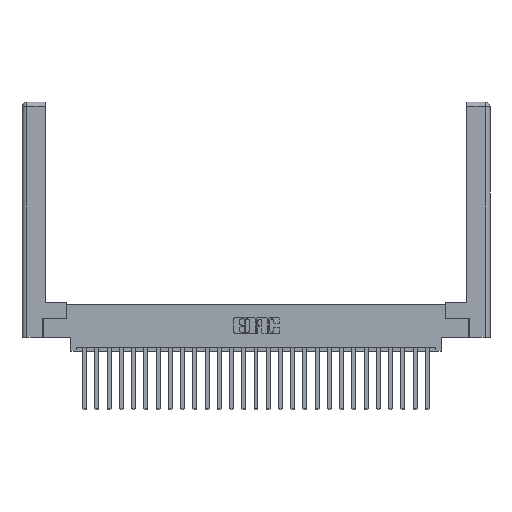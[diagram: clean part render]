
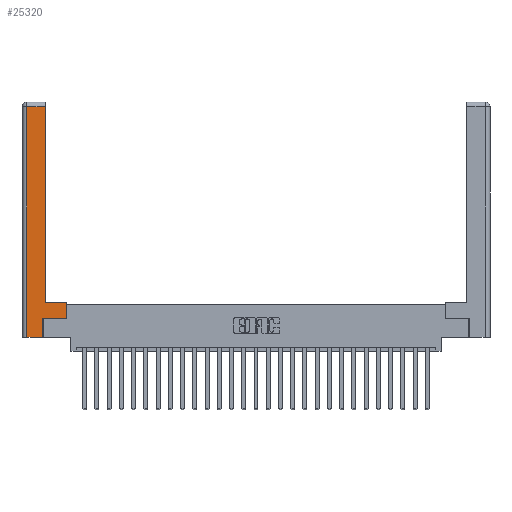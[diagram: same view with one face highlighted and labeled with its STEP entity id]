
A CAD part, top view. The second image highlights one B-rep face of the part: STEP entity #25320.
In plain terms, the highlighted planar face has unit normal (0, 0, 1).
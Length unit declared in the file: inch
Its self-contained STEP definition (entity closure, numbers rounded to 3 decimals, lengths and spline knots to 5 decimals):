
#181 = ORIENTED_EDGE ( 'NONE', *, *, #18120, .T. ) ;
#183 = CARTESIAN_POINT ( 'NONE',  ( 0.565, 0.245, 0. ) ) ;
#653 = LINE ( 'NONE', #11750, #4241 ) ;
#1042 = CARTESIAN_POINT ( 'NONE',  ( 0.265, 0., 0. ) ) ;
#1676 = LINE ( 'NONE', #9965, #18192 ) ;
#2169 = VERTEX_POINT ( 'NONE', #183 ) ;
#3119 = CARTESIAN_POINT ( 'NONE',  ( 0.295, 0.45, 0. ) ) ;
#4077 = ORIENTED_EDGE ( 'NONE', *, *, #25276, .T. ) ;
#4241 = VECTOR ( 'NONE', #21911, 39.37008 ) ;
#4750 = FACE_OUTER_BOUND ( 'NONE', #24954, .T. ) ;
#4895 = VECTOR ( 'NONE', #6860, 39.37008 ) ;
#5386 = CARTESIAN_POINT ( 'NONE',  ( 0.295, 0.45, 0. ) ) ;
#5561 = EDGE_CURVE ( 'NONE', #22152, #10963, #23265, .T. ) ;
#5761 = ORIENTED_EDGE ( 'NONE', *, *, #18331, .T. ) ;
#5882 = EDGE_CURVE ( 'NONE', #16050, #10681, #653, .T. ) ;
#6171 = VECTOR ( 'NONE', #11634, 39.37008 ) ;
#6860 = DIRECTION ( 'NONE',  ( 0., 1., 0. ) ) ;
#7297 = CARTESIAN_POINT ( 'NONE',  ( 0.265, 0.245, 0. ) ) ;
#7337 = ORIENTED_EDGE ( 'NONE', *, *, #5882, .T. ) ;
#7448 = VERTEX_POINT ( 'NONE', #13748 ) ;
#7829 = DIRECTION ( 'NONE',  ( 0., -1., 0. ) ) ;
#8129 = LINE ( 'NONE', #21230, #21371 ) ;
#8367 = AXIS2_PLACEMENT_3D ( 'NONE', #10323, #26649, #16479 ) ;
#8398 = DIRECTION ( 'NONE',  ( 1., 0., 0. ) ) ;
#8444 = CARTESIAN_POINT ( 'NONE',  ( 0.0615, 2.94, 0. ) ) ;
#9965 = CARTESIAN_POINT ( 'NONE',  ( 0.0615, 0., 0. ) ) ;
#10054 = PLANE ( 'NONE',  #8367 ) ;
#10323 = CARTESIAN_POINT ( 'NONE',  ( 0., 0., 0. ) ) ;
#10681 = VERTEX_POINT ( 'NONE', #16983 ) ;
#10720 = ORIENTED_EDGE ( 'NONE', *, *, #5561, .T. ) ;
#10963 = VERTEX_POINT ( 'NONE', #7297 ) ;
#11634 = DIRECTION ( 'NONE',  ( 0., 1., 0. ) ) ;
#11750 = CARTESIAN_POINT ( 'NONE',  ( 0.295, 3., 0. ) ) ;
#13748 = CARTESIAN_POINT ( 'NONE',  ( 0.0615, 0., 0. ) ) ;
#14403 = DIRECTION ( 'NONE',  ( -1., 0., 0. ) ) ;
#15169 = DIRECTION ( 'NONE',  ( 1., 0., 0. ) ) ;
#16050 = VERTEX_POINT ( 'NONE', #5386 ) ;
#16479 = DIRECTION ( 'NONE',  ( -1., 0., 0. ) ) ;
#16523 = CARTESIAN_POINT ( 'NONE',  ( 0.265, 0., 0. ) ) ;
#16851 = CARTESIAN_POINT ( 'NONE',  ( 0.0615, 2.94, 0. ) ) ;
#16983 = CARTESIAN_POINT ( 'NONE',  ( 0.295, 2.94, 0. ) ) ;
#17135 = CARTESIAN_POINT ( 'NONE',  ( 0.565, 0.45, 0. ) ) ;
#17183 = LINE ( 'NONE', #16523, #24277 ) ;
#17530 = VECTOR ( 'NONE', #26356, 39.37008 ) ;
#18120 = EDGE_CURVE ( 'NONE', #7448, #22152, #17183, .T. ) ;
#18161 = LINE ( 'NONE', #3119, #17530 ) ;
#18192 = VECTOR ( 'NONE', #7829, 39.37008 ) ;
#18331 = EDGE_CURVE ( 'NONE', #22255, #16050, #18161, .T. ) ;
#18707 = EDGE_CURVE ( 'NONE', #2169, #22255, #22301, .T. ) ;
#19498 = VECTOR ( 'NONE', #14403, 39.37008 ) ;
#19935 = CARTESIAN_POINT ( 'NONE',  ( 0.265, 0.245, 0. ) ) ;
#19993 = EDGE_CURVE ( 'NONE', #10681, #21200, #22020, .T. ) ;
#20684 = EDGE_CURVE ( 'NONE', #10963, #2169, #8129, .T. ) ;
#21200 = VERTEX_POINT ( 'NONE', #16851 ) ;
#21230 = CARTESIAN_POINT ( 'NONE',  ( 0.565, 0.245, 0. ) ) ;
#21371 = VECTOR ( 'NONE', #15169, 39.37008 ) ;
#21911 = DIRECTION ( 'NONE',  ( 0., 1., 0. ) ) ;
#22020 = LINE ( 'NONE', #8444, #19498 ) ;
#22152 = VERTEX_POINT ( 'NONE', #1042 ) ;
#22255 = VERTEX_POINT ( 'NONE', #23902 ) ;
#22301 = LINE ( 'NONE', #17135, #4895 ) ;
#23152 = ORIENTED_EDGE ( 'NONE', *, *, #19993, .T. ) ;
#23265 = LINE ( 'NONE', #19935, #6171 ) ;
#23902 = CARTESIAN_POINT ( 'NONE',  ( 0.565, 0.45, 0. ) ) ;
#24277 = VECTOR ( 'NONE', #8398, 39.37008 ) ;
#24361 = ORIENTED_EDGE ( 'NONE', *, *, #18707, .T. ) ;
#24954 = EDGE_LOOP ( 'NONE', ( #7337, #23152, #4077, #181, #10720, #26470, #24361, #5761 ) ) ;
#25276 = EDGE_CURVE ( 'NONE', #21200, #7448, #1676, .T. ) ;
#25320 = ADVANCED_FACE ( 'NONE', ( #4750 ), #10054, .F. ) ;
#26356 = DIRECTION ( 'NONE',  ( -1., 0., 0. ) ) ;
#26470 = ORIENTED_EDGE ( 'NONE', *, *, #20684, .T. ) ;
#26649 = DIRECTION ( 'NONE',  ( 0., 0., -1. ) ) ;
